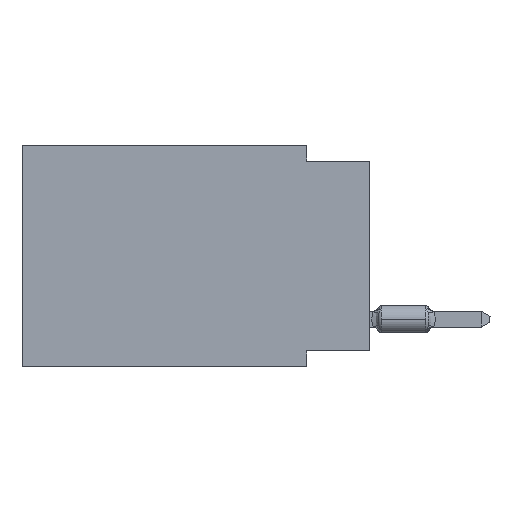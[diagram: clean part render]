
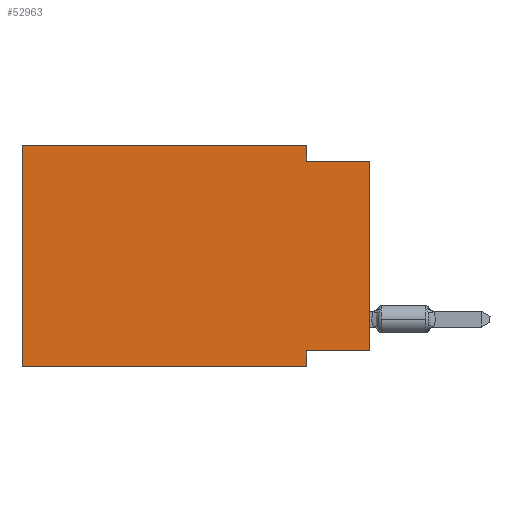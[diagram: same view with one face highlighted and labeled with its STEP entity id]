
A CAD part, left-side view. The second image highlights one B-rep face of the part: STEP entity #52963.
In plain terms, the highlighted planar face has unit normal (-1, 0, 0).
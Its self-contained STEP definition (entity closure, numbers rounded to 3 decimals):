
#662 = CARTESIAN_POINT ( 'NONE',  ( 0., 13.97, 0. ) ) ;
#2220 = VERTEX_POINT ( 'NONE', #58818 ) ;
#3196 = EDGE_LOOP ( 'NONE', ( #66065, #48405, #48175, #32015, #21785, #33012, #24416, #24319 ) ) ;
#3429 = DIRECTION ( 'NONE',  ( 0., 0., -1. ) ) ;
#4408 = VERTEX_POINT ( 'NONE', #24643 ) ;
#4639 = LINE ( 'NONE', #47599, #23828 ) ;
#5001 = CARTESIAN_POINT ( 'NONE',  ( 0., 13.97, -8.89 ) ) ;
#5381 = VECTOR ( 'NONE', #27213, 1000. ) ;
#5382 = EDGE_CURVE ( 'NONE', #2220, #16383, #28960, .T. ) ;
#9801 = CARTESIAN_POINT ( 'NONE',  ( 0., 0., -8.255 ) ) ;
#10779 = VECTOR ( 'NONE', #26307, 1000. ) ;
#14010 = CARTESIAN_POINT ( 'NONE',  ( 0., 13.97, -8.89 ) ) ;
#15401 = DIRECTION ( 'NONE',  ( 0., -1., 0. ) ) ;
#16383 = VERTEX_POINT ( 'NONE', #67200 ) ;
#17039 = LINE ( 'NONE', #38849, #26466 ) ;
#20025 = EDGE_CURVE ( 'NONE', #68527, #29309, #50832, .T. ) ;
#20997 = EDGE_CURVE ( 'NONE', #68527, #4408, #37016, .T. ) ;
#21785 = ORIENTED_EDGE ( 'NONE', *, *, #64898, .F. ) ;
#22306 = VECTOR ( 'NONE', #38978, 1000. ) ;
#22825 = CARTESIAN_POINT ( 'NONE',  ( 0., 2.54, -8.89 ) ) ;
#23828 = VECTOR ( 'NONE', #15401, 1000. ) ;
#24319 = ORIENTED_EDGE ( 'NONE', *, *, #20997, .F. ) ;
#24416 = ORIENTED_EDGE ( 'NONE', *, *, #38889, .F. ) ;
#24643 = CARTESIAN_POINT ( 'NONE',  ( 0., 2.54, -8.255 ) ) ;
#26307 = DIRECTION ( 'NONE',  ( 0., 1., 0. ) ) ;
#26466 = VECTOR ( 'NONE', #60722, 1000. ) ;
#27213 = DIRECTION ( 'NONE',  ( 0., -1., 0. ) ) ;
#28960 = LINE ( 'NONE', #662, #22306 ) ;
#29309 = VERTEX_POINT ( 'NONE', #31976 ) ;
#29597 = LINE ( 'NONE', #22825, #62255 ) ;
#31976 = CARTESIAN_POINT ( 'NONE',  ( 0., 0., -0.635 ) ) ;
#32015 = ORIENTED_EDGE ( 'NONE', *, *, #5382, .F. ) ;
#32642 = VERTEX_POINT ( 'NONE', #14010 ) ;
#33012 = ORIENTED_EDGE ( 'NONE', *, *, #61692, .T. ) ;
#34017 = DIRECTION ( 'NONE',  ( 0., 0., 1. ) ) ;
#34241 = DIRECTION ( 'NONE',  ( 0., 0., -1. ) ) ;
#35212 = VERTEX_POINT ( 'NONE', #49633 ) ;
#36006 = LINE ( 'NONE', #57870, #65054 ) ;
#36229 = AXIS2_PLACEMENT_3D ( 'NONE', #59970, #55297, #44198 ) ;
#37016 = LINE ( 'NONE', #9801, #10779 ) ;
#38849 = CARTESIAN_POINT ( 'NONE',  ( 0., 13.97, 0. ) ) ;
#38889 = EDGE_CURVE ( 'NONE', #4408, #65658, #29597, .T. ) ;
#38978 = DIRECTION ( 'NONE',  ( 0., -1., 0. ) ) ;
#43299 = LINE ( 'NONE', #5001, #5381 ) ;
#44198 = DIRECTION ( 'NONE',  ( 0., 0., -1. ) ) ;
#47599 = CARTESIAN_POINT ( 'NONE',  ( 0., 0., -0.635 ) ) ;
#48175 = ORIENTED_EDGE ( 'NONE', *, *, #49268, .F. ) ;
#48405 = ORIENTED_EDGE ( 'NONE', *, *, #67164, .F. ) ;
#49219 = FACE_OUTER_BOUND ( 'NONE', #3196, .T. ) ;
#49268 = EDGE_CURVE ( 'NONE', #16383, #35212, #36006, .T. ) ;
#49633 = CARTESIAN_POINT ( 'NONE',  ( 0., 2.54, -0.635 ) ) ;
#50832 = LINE ( 'NONE', #51186, #58061 ) ;
#51186 = CARTESIAN_POINT ( 'NONE',  ( 0., 0., 0. ) ) ;
#52963 = ADVANCED_FACE ( 'NONE', ( #49219 ), #60320, .F. ) ;
#55297 = DIRECTION ( 'NONE',  ( 1., 0., 0. ) ) ;
#56784 = CARTESIAN_POINT ( 'NONE',  ( 0., 0., -8.255 ) ) ;
#57870 = CARTESIAN_POINT ( 'NONE',  ( 0., 2.54, 0. ) ) ;
#58061 = VECTOR ( 'NONE', #34017, 1000. ) ;
#58818 = CARTESIAN_POINT ( 'NONE',  ( 0., 13.97, 0. ) ) ;
#59970 = CARTESIAN_POINT ( 'NONE',  ( 0., 13.97, 0. ) ) ;
#60320 = PLANE ( 'NONE',  #36229 ) ;
#60722 = DIRECTION ( 'NONE',  ( 0., 0., 1. ) ) ;
#61692 = EDGE_CURVE ( 'NONE', #32642, #65658, #43299, .T. ) ;
#62255 = VECTOR ( 'NONE', #34241, 1000. ) ;
#64898 = EDGE_CURVE ( 'NONE', #32642, #2220, #17039, .T. ) ;
#65054 = VECTOR ( 'NONE', #3429, 1000. ) ;
#65230 = CARTESIAN_POINT ( 'NONE',  ( 0., 2.54, -8.89 ) ) ;
#65658 = VERTEX_POINT ( 'NONE', #65230 ) ;
#66065 = ORIENTED_EDGE ( 'NONE', *, *, #20025, .T. ) ;
#67164 = EDGE_CURVE ( 'NONE', #35212, #29309, #4639, .T. ) ;
#67200 = CARTESIAN_POINT ( 'NONE',  ( 0., 2.54, 0. ) ) ;
#68527 = VERTEX_POINT ( 'NONE', #56784 ) ;
